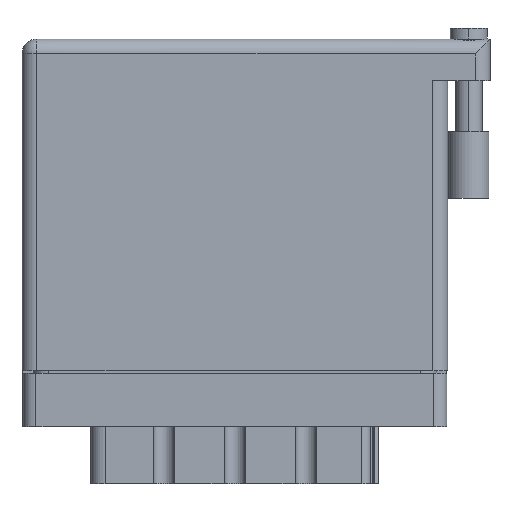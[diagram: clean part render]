
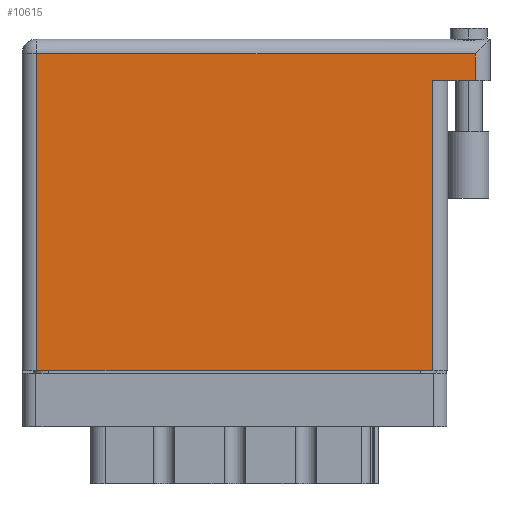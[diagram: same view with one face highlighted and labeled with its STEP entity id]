
A CAD part, front view. The second image highlights one B-rep face of the part: STEP entity #10615.
In plain terms, the highlighted face is planar.
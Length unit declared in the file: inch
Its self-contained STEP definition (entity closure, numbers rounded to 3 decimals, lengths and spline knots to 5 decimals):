
#32 = CARTESIAN_POINT ( 'NONE',  ( 0.07, 0., 0. ) ) ;
#2959 = CARTESIAN_POINT ( 'NONE',  ( 2.138, 1.496, 0. ) ) ;
#4173 = CARTESIAN_POINT ( 'NONE',  ( 1.938, 1.369, 0. ) ) ;
#4682 = VECTOR ( 'NONE', #18487, 39.37008 ) ;
#4684 = PLANE ( 'NONE',  #30805 ) ;
#4687 = FACE_OUTER_BOUND ( 'NONE', #14494, .T. ) ;
#4819 = EDGE_CURVE ( 'NONE', #23025, #28559, #24281, .T. ) ;
#4890 = EDGE_CURVE ( 'NONE', #17950, #20743, #26081, .T. ) ;
#7119 = ORIENTED_EDGE ( 'NONE', *, *, #32449, .T. ) ;
#7231 = CARTESIAN_POINT ( 'NONE',  ( 0., 1.496, 0. ) ) ;
#7555 = CARTESIAN_POINT ( 'NONE',  ( 0., 1.566, 0. ) ) ;
#7647 = DIRECTION ( 'NONE',  ( 0., -1., 0. ) ) ;
#7746 = ORIENTED_EDGE ( 'NONE', *, *, #23835, .T. ) ;
#8419 = CARTESIAN_POINT ( 'NONE',  ( 2.208, 1.369, 0. ) ) ;
#9352 = LINE ( 'NONE', #8419, #31185 ) ;
#10572 = CARTESIAN_POINT ( 'NONE',  ( 2.138, 1.369, 0. ) ) ;
#10615 = ADVANCED_FACE ( 'NONE', ( #4687 ), #4684, .F. ) ;
#11106 = EDGE_CURVE ( 'NONE', #20743, #23025, #17577, .T. ) ;
#14148 = DIRECTION ( 'NONE',  ( -1., 0., 0. ) ) ;
#14494 = EDGE_LOOP ( 'NONE', ( #20944, #17271, #26989, #7119, #7746, #14921 ) ) ;
#14921 = ORIENTED_EDGE ( 'NONE', *, *, #4890, .T. ) ;
#15202 = LINE ( 'NONE', #23787, #27663 ) ;
#15220 = DIRECTION ( 'NONE',  ( 0., 1., 0. ) ) ;
#15810 = DIRECTION ( 'NONE',  ( 0., 0., -1. ) ) ;
#16709 = CARTESIAN_POINT ( 'NONE',  ( 1.938, 1.369, 0. ) ) ;
#17271 = ORIENTED_EDGE ( 'NONE', *, *, #4819, .T. ) ;
#17577 = LINE ( 'NONE', #27417, #24251 ) ;
#17950 = VERTEX_POINT ( 'NONE', #29519 ) ;
#18261 = VERTEX_POINT ( 'NONE', #2959 ) ;
#18487 = DIRECTION ( 'NONE',  ( 0., 1., 0. ) ) ;
#19602 = EDGE_CURVE ( 'NONE', #22801, #28559, #9352, .T. ) ;
#20743 = VERTEX_POINT ( 'NONE', #32 ) ;
#20944 = ORIENTED_EDGE ( 'NONE', *, *, #11106, .T. ) ;
#22801 = VERTEX_POINT ( 'NONE', #10572 ) ;
#23025 = VERTEX_POINT ( 'NONE', #23236 ) ;
#23236 = CARTESIAN_POINT ( 'NONE',  ( 1.938, 0., 0. ) ) ;
#23787 = CARTESIAN_POINT ( 'NONE',  ( 2.138, 1.566, 0. ) ) ;
#23835 = EDGE_CURVE ( 'NONE', #18261, #17950, #30403, .T. ) ;
#24187 = DIRECTION ( 'NONE',  ( -1., 0., 0. ) ) ;
#24251 = VECTOR ( 'NONE', #35734, 39.37008 ) ;
#24281 = LINE ( 'NONE', #4173, #4682 ) ;
#24712 = CARTESIAN_POINT ( 'NONE',  ( 0.07, 0., 0. ) ) ;
#26081 = LINE ( 'NONE', #24712, #26540 ) ;
#26540 = VECTOR ( 'NONE', #7647, 39.37008 ) ;
#26989 = ORIENTED_EDGE ( 'NONE', *, *, #19602, .F. ) ;
#27417 = CARTESIAN_POINT ( 'NONE',  ( 0., 0., 0. ) ) ;
#27501 = DIRECTION ( 'NONE',  ( -1., 0., 0. ) ) ;
#27663 = VECTOR ( 'NONE', #15220, 39.37008 ) ;
#28559 = VERTEX_POINT ( 'NONE', #16709 ) ;
#29519 = CARTESIAN_POINT ( 'NONE',  ( 0.07, 1.496, 0. ) ) ;
#30403 = LINE ( 'NONE', #7231, #33037 ) ;
#30805 = AXIS2_PLACEMENT_3D ( 'NONE', #7555, #15810, #27501 ) ;
#31185 = VECTOR ( 'NONE', #14148, 39.37008 ) ;
#32449 = EDGE_CURVE ( 'NONE', #22801, #18261, #15202, .T. ) ;
#33037 = VECTOR ( 'NONE', #24187, 39.37008 ) ;
#35734 = DIRECTION ( 'NONE',  ( 1., 0., 0. ) ) ;
